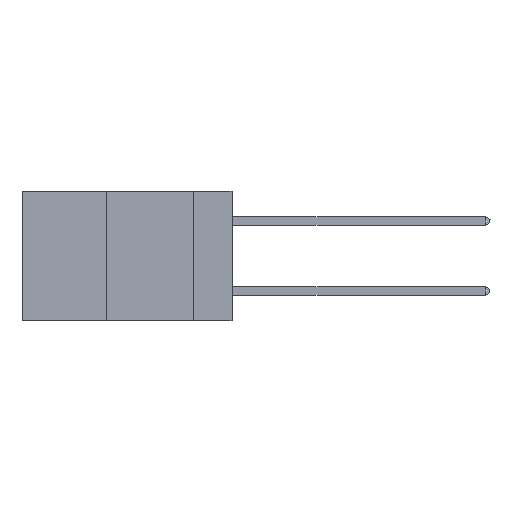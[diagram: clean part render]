
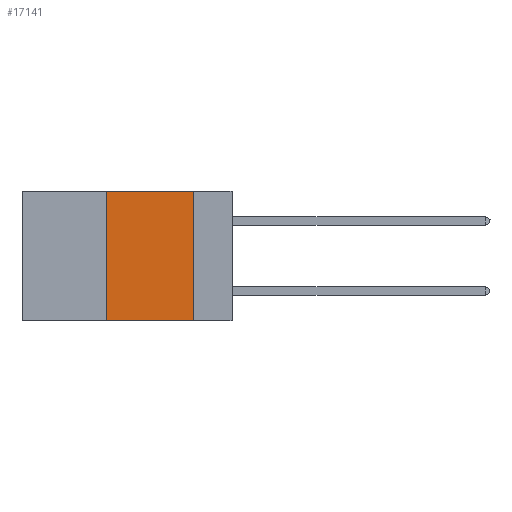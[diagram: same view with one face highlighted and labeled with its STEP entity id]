
A CAD part, left-side view. The second image highlights one B-rep face of the part: STEP entity #17141.
In plain terms, the highlighted planar face has unit normal (-1, 0, 0).
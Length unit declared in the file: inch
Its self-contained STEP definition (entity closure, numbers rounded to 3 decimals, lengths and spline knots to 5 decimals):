
#37 = EDGE_CURVE ( 'NONE', #19172, #8731, #6795, .T. ) ;
#508 = LINE ( 'NONE', #11998, #7585 ) ;
#585 = EDGE_CURVE ( 'NONE', #18959, #8731, #4347, .T. ) ;
#727 = EDGE_CURVE ( 'NONE', #19172, #794, #12138, .T. ) ;
#794 = VERTEX_POINT ( 'NONE', #10129 ) ;
#1583 = VECTOR ( 'NONE', #12457, 39.37008 ) ;
#2170 = CARTESIAN_POINT ( 'NONE',  ( 0., 0.36, 0. ) ) ;
#2404 = ORIENTED_EDGE ( 'NONE', *, *, #585, .F. ) ;
#2980 = EDGE_CURVE ( 'NONE', #794, #18959, #508, .T. ) ;
#3950 = CARTESIAN_POINT ( 'NONE',  ( 0., 0.11, 0. ) ) ;
#4347 = LINE ( 'NONE', #14816, #17795 ) ;
#4485 = VECTOR ( 'NONE', #23724, 39.37008 ) ;
#5436 = FACE_OUTER_BOUND ( 'NONE', #21833, .T. ) ;
#5968 = DIRECTION ( 'NONE',  ( 0., 0., -1. ) ) ;
#6795 = LINE ( 'NONE', #18254, #1583 ) ;
#7585 = VECTOR ( 'NONE', #18377, 39.37008 ) ;
#8731 = VERTEX_POINT ( 'NONE', #19612 ) ;
#10071 = DIRECTION ( 'NONE',  ( 1., 0., 0. ) ) ;
#10129 = CARTESIAN_POINT ( 'NONE',  ( 0., 0.36, 0. ) ) ;
#10203 = ORIENTED_EDGE ( 'NONE', *, *, #37, .T. ) ;
#11998 = CARTESIAN_POINT ( 'NONE',  ( 0., 0.6, 0. ) ) ;
#12138 = LINE ( 'NONE', #2170, #4485 ) ;
#12457 = DIRECTION ( 'NONE',  ( 0., -1., 0. ) ) ;
#12850 = DIRECTION ( 'NONE',  ( 0., 0., -1. ) ) ;
#13421 = AXIS2_PLACEMENT_3D ( 'NONE', #17670, #10071, #5968 ) ;
#14816 = CARTESIAN_POINT ( 'NONE',  ( 0., 0.11, 0. ) ) ;
#15049 = ORIENTED_EDGE ( 'NONE', *, *, #2980, .F. ) ;
#16352 = ORIENTED_EDGE ( 'NONE', *, *, #727, .F. ) ;
#16924 = CARTESIAN_POINT ( 'NONE',  ( 0., 0.36, -0.37 ) ) ;
#17141 = ADVANCED_FACE ( 'NONE', ( #5436 ), #23390, .F. ) ;
#17670 = CARTESIAN_POINT ( 'NONE',  ( 0., 0.6, 0. ) ) ;
#17795 = VECTOR ( 'NONE', #12850, 39.37008 ) ;
#18254 = CARTESIAN_POINT ( 'NONE',  ( 0., 0.6, -0.37 ) ) ;
#18377 = DIRECTION ( 'NONE',  ( 0., -1., 0. ) ) ;
#18959 = VERTEX_POINT ( 'NONE', #3950 ) ;
#19172 = VERTEX_POINT ( 'NONE', #16924 ) ;
#19612 = CARTESIAN_POINT ( 'NONE',  ( 0., 0.11, -0.37 ) ) ;
#21833 = EDGE_LOOP ( 'NONE', ( #2404, #15049, #16352, #10203 ) ) ;
#23390 = PLANE ( 'NONE',  #13421 ) ;
#23724 = DIRECTION ( 'NONE',  ( 0., 0., 1. ) ) ;
